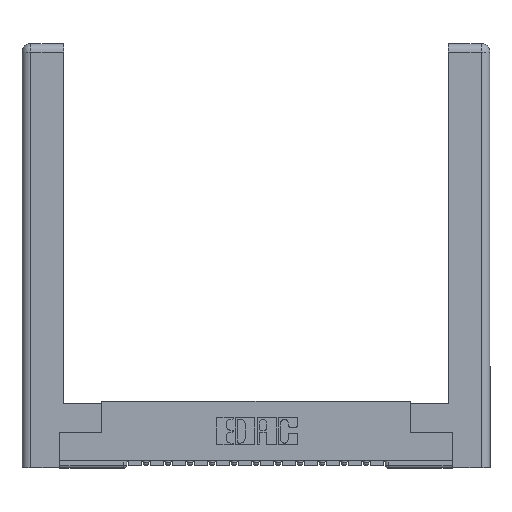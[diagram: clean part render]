
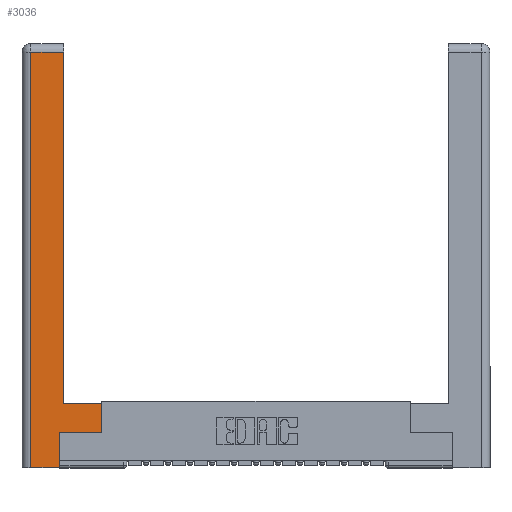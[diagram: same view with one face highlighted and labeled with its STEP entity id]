
A CAD part, top view. The second image highlights one B-rep face of the part: STEP entity #3036.
In plain terms, the highlighted planar face has unit normal (0, 0, 1).
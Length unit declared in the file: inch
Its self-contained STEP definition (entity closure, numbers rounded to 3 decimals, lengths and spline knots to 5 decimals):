
#746 = VERTEX_POINT ( 'NONE', #6992 ) ;
#915 = CARTESIAN_POINT ( 'NONE',  ( 0., 0., 0. ) ) ;
#1511 = VERTEX_POINT ( 'NONE', #13102 ) ;
#1544 = LINE ( 'NONE', #12506, #3567 ) ;
#1702 = LINE ( 'NONE', #7143, #10879 ) ;
#1808 = CARTESIAN_POINT ( 'NONE',  ( 0.565, 0.245, 0. ) ) ;
#1973 = CARTESIAN_POINT ( 'NONE',  ( 0.565, 0.45, 0. ) ) ;
#2179 = VERTEX_POINT ( 'NONE', #9869 ) ;
#2375 = CARTESIAN_POINT ( 'NONE',  ( 0.265, 0.245, 0. ) ) ;
#3036 = ADVANCED_FACE ( 'NONE', ( #9114 ), #14645, .F. ) ;
#3115 = CARTESIAN_POINT ( 'NONE',  ( 0.565, 0.245, 0. ) ) ;
#3210 = DIRECTION ( 'NONE',  ( -1., 0., 0. ) ) ;
#3372 = LINE ( 'NONE', #8984, #11508 ) ;
#3567 = VECTOR ( 'NONE', #5554, 39.37008 ) ;
#3684 = ORIENTED_EDGE ( 'NONE', *, *, #9590, .T. ) ;
#4583 = CARTESIAN_POINT ( 'NONE',  ( 0.0615, 0., 0. ) ) ;
#5554 = DIRECTION ( 'NONE',  ( -1., 0., 0. ) ) ;
#5583 = ORIENTED_EDGE ( 'NONE', *, *, #13814, .T. ) ;
#5923 = CARTESIAN_POINT ( 'NONE',  ( 0.295, 2.94, 0. ) ) ;
#6158 = LINE ( 'NONE', #1973, #14238 ) ;
#6510 = VERTEX_POINT ( 'NONE', #14649 ) ;
#6604 = ORIENTED_EDGE ( 'NONE', *, *, #12669, .T. ) ;
#6810 = LINE ( 'NONE', #7796, #14838 ) ;
#6992 = CARTESIAN_POINT ( 'NONE',  ( 0.565, 0.45, 0. ) ) ;
#7143 = CARTESIAN_POINT ( 'NONE',  ( 0.0615, 2.94, 0. ) ) ;
#7536 = ORIENTED_EDGE ( 'NONE', *, *, #8377, .T. ) ;
#7752 = VERTEX_POINT ( 'NONE', #2375 ) ;
#7796 = CARTESIAN_POINT ( 'NONE',  ( 0.295, 3., 0. ) ) ;
#7964 = EDGE_CURVE ( 'NONE', #1511, #12943, #8851, .T. ) ;
#8055 = DIRECTION ( 'NONE',  ( -1., 0., 0. ) ) ;
#8243 = VERTEX_POINT ( 'NONE', #3115 ) ;
#8377 = EDGE_CURVE ( 'NONE', #12943, #6510, #3372, .T. ) ;
#8578 = VECTOR ( 'NONE', #15186, 39.37008 ) ;
#8851 = LINE ( 'NONE', #4583, #16891 ) ;
#8984 = CARTESIAN_POINT ( 'NONE',  ( 0.265, 0., 0. ) ) ;
#9114 = FACE_OUTER_BOUND ( 'NONE', #13589, .T. ) ;
#9566 = LINE ( 'NONE', #1808, #8578 ) ;
#9590 = EDGE_CURVE ( 'NONE', #746, #2179, #1544, .T. ) ;
#9869 = CARTESIAN_POINT ( 'NONE',  ( 0.295, 0.45, 0. ) ) ;
#10494 = ORIENTED_EDGE ( 'NONE', *, *, #7964, .T. ) ;
#10879 = VECTOR ( 'NONE', #3210, 39.37008 ) ;
#11190 = VECTOR ( 'NONE', #17408, 39.37008 ) ;
#11508 = VECTOR ( 'NONE', #15766, 39.37008 ) ;
#12196 = VERTEX_POINT ( 'NONE', #5923 ) ;
#12506 = CARTESIAN_POINT ( 'NONE',  ( 0.295, 0.45, 0. ) ) ;
#12622 = ORIENTED_EDGE ( 'NONE', *, *, #16226, .T. ) ;
#12669 = EDGE_CURVE ( 'NONE', #8243, #746, #6158, .T. ) ;
#12943 = VERTEX_POINT ( 'NONE', #14900 ) ;
#13102 = CARTESIAN_POINT ( 'NONE',  ( 0.0615, 2.94, 0. ) ) ;
#13235 = CARTESIAN_POINT ( 'NONE',  ( 0.265, 0.245, 0. ) ) ;
#13575 = ORIENTED_EDGE ( 'NONE', *, *, #13696, .T. ) ;
#13589 = EDGE_LOOP ( 'NONE', ( #13575, #12622, #10494, #7536, #15906, #5583, #6604, #3684 ) ) ;
#13590 = LINE ( 'NONE', #13235, #11190 ) ;
#13696 = EDGE_CURVE ( 'NONE', #2179, #12196, #6810, .T. ) ;
#13814 = EDGE_CURVE ( 'NONE', #7752, #8243, #9566, .T. ) ;
#13949 = DIRECTION ( 'NONE',  ( 0., -1., 0. ) ) ;
#14238 = VECTOR ( 'NONE', #15697, 39.37008 ) ;
#14645 = PLANE ( 'NONE',  #17041 ) ;
#14649 = CARTESIAN_POINT ( 'NONE',  ( 0.265, 0., 0. ) ) ;
#14838 = VECTOR ( 'NONE', #16251, 39.37008 ) ;
#14900 = CARTESIAN_POINT ( 'NONE',  ( 0.0615, 0., 0. ) ) ;
#15186 = DIRECTION ( 'NONE',  ( 1., 0., 0. ) ) ;
#15697 = DIRECTION ( 'NONE',  ( 0., 1., 0. ) ) ;
#15766 = DIRECTION ( 'NONE',  ( 1., 0., 0. ) ) ;
#15906 = ORIENTED_EDGE ( 'NONE', *, *, #17288, .T. ) ;
#16069 = DIRECTION ( 'NONE',  ( 0., 0., -1. ) ) ;
#16226 = EDGE_CURVE ( 'NONE', #12196, #1511, #1702, .T. ) ;
#16251 = DIRECTION ( 'NONE',  ( 0., 1., 0. ) ) ;
#16891 = VECTOR ( 'NONE', #13949, 39.37008 ) ;
#17041 = AXIS2_PLACEMENT_3D ( 'NONE', #915, #16069, #8055 ) ;
#17288 = EDGE_CURVE ( 'NONE', #6510, #7752, #13590, .T. ) ;
#17408 = DIRECTION ( 'NONE',  ( 0., 1., 0. ) ) ;
